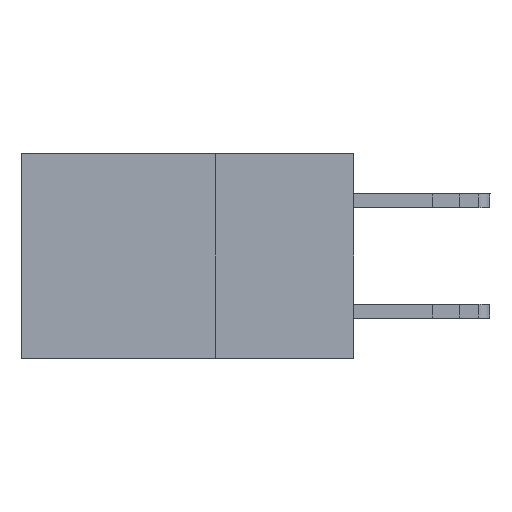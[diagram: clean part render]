
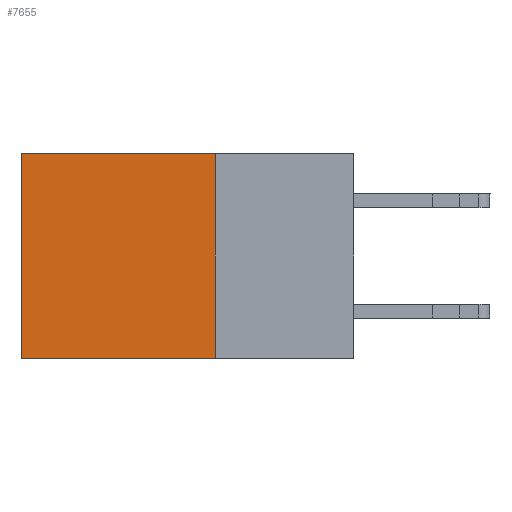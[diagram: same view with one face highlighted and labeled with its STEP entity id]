
A CAD part, left-side view. The second image highlights one B-rep face of the part: STEP entity #7655.
In plain terms, the highlighted planar face has unit normal (-1, 0, 0).
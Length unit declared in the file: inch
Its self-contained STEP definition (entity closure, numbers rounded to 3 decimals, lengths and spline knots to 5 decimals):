
#1771 = CARTESIAN_POINT ( 'NONE',  ( 0.2875, 0.25, 0. ) ) ;
#2363 = EDGE_CURVE ( 'NONE', #16771, #6055, #26945, .T. ) ;
#4138 = LINE ( 'NONE', #6112, #28416 ) ;
#4146 = VECTOR ( 'NONE', #5006, 39.37008 ) ;
#5006 = DIRECTION ( 'NONE',  ( 0., 1., 0. ) ) ;
#5130 = FACE_OUTER_BOUND ( 'NONE', #12709, .T. ) ;
#5149 = LINE ( 'NONE', #15076, #29439 ) ;
#6055 = VERTEX_POINT ( 'NONE', #30117 ) ;
#6112 = CARTESIAN_POINT ( 'NONE',  ( 0.2875, 0.6, 0. ) ) ;
#6572 = ORIENTED_EDGE ( 'NONE', *, *, #23888, .F. ) ;
#7655 = ADVANCED_FACE ( 'NONE', ( #5130 ), #30458, .F. ) ;
#7919 = VERTEX_POINT ( 'NONE', #18163 ) ;
#10146 = VERTEX_POINT ( 'NONE', #13569 ) ;
#10653 = VECTOR ( 'NONE', #11007, 39.37008 ) ;
#11007 = DIRECTION ( 'NONE',  ( 0., 1., 0. ) ) ;
#11058 = ORIENTED_EDGE ( 'NONE', *, *, #17969, .T. ) ;
#12709 = EDGE_LOOP ( 'NONE', ( #11058, #16958, #6572, #28975 ) ) ;
#12746 = DIRECTION ( 'NONE',  ( 0., 0., -1. ) ) ;
#13569 = CARTESIAN_POINT ( 'NONE',  ( 0.2875, 0.6, -0.37 ) ) ;
#15076 = CARTESIAN_POINT ( 'NONE',  ( 0.2875, 0.25, 0. ) ) ;
#16316 = EDGE_CURVE ( 'NONE', #7919, #10146, #29669, .T. ) ;
#16771 = VERTEX_POINT ( 'NONE', #23377 ) ;
#16958 = ORIENTED_EDGE ( 'NONE', *, *, #16316, .F. ) ;
#17969 = EDGE_CURVE ( 'NONE', #6055, #10146, #4138, .T. ) ;
#18163 = CARTESIAN_POINT ( 'NONE',  ( 0.2875, 0.25, -0.37 ) ) ;
#20347 = CARTESIAN_POINT ( 'NONE',  ( 0.2875, 0.25, -0.37 ) ) ;
#20887 = DIRECTION ( 'NONE',  ( 1., 0., 0. ) ) ;
#23377 = CARTESIAN_POINT ( 'NONE',  ( 0.2875, 0.25, 0. ) ) ;
#23888 = EDGE_CURVE ( 'NONE', #16771, #7919, #5149, .T. ) ;
#26414 = CARTESIAN_POINT ( 'NONE',  ( 0.2875, 0.25, 0. ) ) ;
#26945 = LINE ( 'NONE', #26414, #4146 ) ;
#28416 = VECTOR ( 'NONE', #30051, 39.37008 ) ;
#28453 = AXIS2_PLACEMENT_3D ( 'NONE', #1771, #20887, #28935 ) ;
#28935 = DIRECTION ( 'NONE',  ( 0., 0., -1. ) ) ;
#28975 = ORIENTED_EDGE ( 'NONE', *, *, #2363, .T. ) ;
#29439 = VECTOR ( 'NONE', #12746, 39.37008 ) ;
#29669 = LINE ( 'NONE', #20347, #10653 ) ;
#30051 = DIRECTION ( 'NONE',  ( 0., 0., -1. ) ) ;
#30117 = CARTESIAN_POINT ( 'NONE',  ( 0.2875, 0.6, 0. ) ) ;
#30458 = PLANE ( 'NONE',  #28453 ) ;
